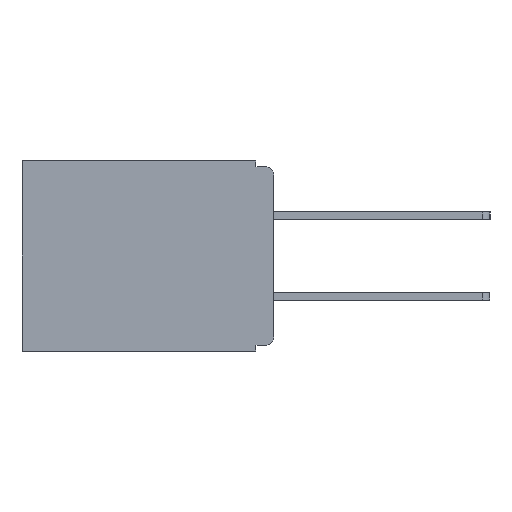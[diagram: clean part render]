
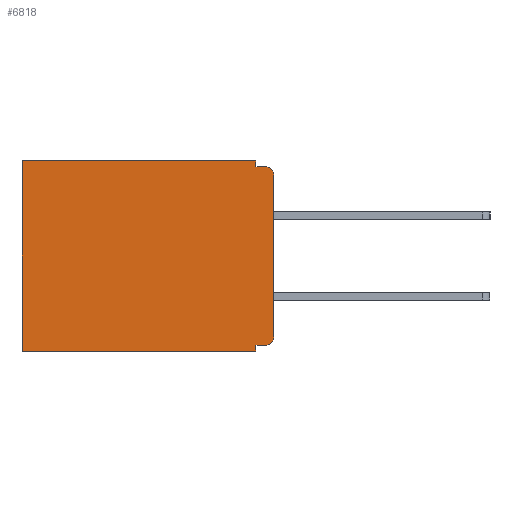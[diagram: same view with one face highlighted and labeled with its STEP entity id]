
A CAD part, left-side view. The second image highlights one B-rep face of the part: STEP entity #6818.
In plain terms, the highlighted planar face has unit normal (-1, 0, 0).
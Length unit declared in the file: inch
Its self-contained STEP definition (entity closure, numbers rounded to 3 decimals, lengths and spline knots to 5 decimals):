
#93 = DIRECTION ( 'NONE',  ( 1., 0., 0. ) ) ;
#342 = VECTOR ( 'NONE', #3753, 39.37008 ) ;
#639 = ORIENTED_EDGE ( 'NONE', *, *, #15581, .T. ) ;
#849 = VECTOR ( 'NONE', #10346, 39.37008 ) ;
#1255 = EDGE_CURVE ( 'NONE', #26265, #23395, #8771, .T. ) ;
#1268 = EDGE_CURVE ( 'NONE', #26265, #24596, #8109, .T. ) ;
#1290 = CARTESIAN_POINT ( 'NONE',  ( 0.3, 0.437, -0.33 ) ) ;
#1765 = VERTEX_POINT ( 'NONE', #7767 ) ;
#1781 = CARTESIAN_POINT ( 'NONE',  ( 0.3, 0.015, -0.305 ) ) ;
#1952 = VERTEX_POINT ( 'NONE', #24529 ) ;
#1975 = ORIENTED_EDGE ( 'NONE', *, *, #1268, .F. ) ;
#1980 = EDGE_CURVE ( 'NONE', #24596, #8565, #9445, .T. ) ;
#2009 = ORIENTED_EDGE ( 'NONE', *, *, #17366, .T. ) ;
#3186 = PLANE ( 'NONE',  #14296 ) ;
#3435 = VERTEX_POINT ( 'NONE', #1290 ) ;
#3664 = VECTOR ( 'NONE', #17647, 39.37008 ) ;
#3705 = DIRECTION ( 'NONE',  ( -1., 0., 0. ) ) ;
#3753 = DIRECTION ( 'NONE',  ( 0., 0., -1. ) ) ;
#4044 = DIRECTION ( 'NONE',  ( 0., 0., -1. ) ) ;
#4134 = VERTEX_POINT ( 'NONE', #11212 ) ;
#4178 = AXIS2_PLACEMENT_3D ( 'NONE', #1781, #16551, #4044 ) ;
#4761 = CARTESIAN_POINT ( 'NONE',  ( 0.3, 0., -0.01 ) ) ;
#4827 = CARTESIAN_POINT ( 'NONE',  ( 0.3, 0.015, -0.32 ) ) ;
#5767 = DIRECTION ( 'NONE',  ( 0., 0., -1. ) ) ;
#6818 = ADVANCED_FACE ( 'NONE', ( #14408 ), #3186, .F. ) ;
#7631 = DIRECTION ( 'NONE',  ( 0., 0., -1. ) ) ;
#7641 = ORIENTED_EDGE ( 'NONE', *, *, #15970, .F. ) ;
#7767 = CARTESIAN_POINT ( 'NONE',  ( 0.3, 0., -0.305 ) ) ;
#8109 = LINE ( 'NONE', #25941, #14249 ) ;
#8565 = VERTEX_POINT ( 'NONE', #25086 ) ;
#8660 = ORIENTED_EDGE ( 'NONE', *, *, #1980, .F. ) ;
#8670 = LINE ( 'NONE', #21833, #18209 ) ;
#8771 = LINE ( 'NONE', #24153, #13592 ) ;
#9291 = LINE ( 'NONE', #22622, #20660 ) ;
#9384 = ORIENTED_EDGE ( 'NONE', *, *, #19107, .F. ) ;
#9434 = ORIENTED_EDGE ( 'NONE', *, *, #25076, .F. ) ;
#9445 = LINE ( 'NONE', #4761, #3664 ) ;
#10346 = DIRECTION ( 'NONE',  ( 0., 1., 0. ) ) ;
#11212 = CARTESIAN_POINT ( 'NONE',  ( 0.3, 0., -0.025 ) ) ;
#11640 = LINE ( 'NONE', #22080, #26401 ) ;
#12965 = ORIENTED_EDGE ( 'NONE', *, *, #14863, .T. ) ;
#13592 = VECTOR ( 'NONE', #25249, 39.37008 ) ;
#14249 = VECTOR ( 'NONE', #25065, 39.37008 ) ;
#14296 = AXIS2_PLACEMENT_3D ( 'NONE', #24427, #93, #7631 ) ;
#14314 = EDGE_CURVE ( 'NONE', #1952, #3435, #17671, .T. ) ;
#14408 = FACE_OUTER_BOUND ( 'NONE', #26288, .T. ) ;
#14529 = CIRCLE ( 'NONE', #15588, 0.015 ) ;
#14863 = EDGE_CURVE ( 'NONE', #4134, #8565, #14529, .T. ) ;
#15581 = EDGE_CURVE ( 'NONE', #17558, #1765, #18234, .T. ) ;
#15588 = AXIS2_PLACEMENT_3D ( 'NONE', #16240, #3705, #18256 ) ;
#15970 = EDGE_CURVE ( 'NONE', #17558, #24839, #8670, .T. ) ;
#16240 = CARTESIAN_POINT ( 'NONE',  ( 0.3, 0.015, -0.025 ) ) ;
#16551 = DIRECTION ( 'NONE',  ( -1., 0., 0. ) ) ;
#17366 = EDGE_CURVE ( 'NONE', #23395, #3435, #9291, .T. ) ;
#17558 = VERTEX_POINT ( 'NONE', #4827 ) ;
#17647 = DIRECTION ( 'NONE',  ( 0., -1., 0. ) ) ;
#17671 = LINE ( 'NONE', #18374, #849 ) ;
#17851 = LINE ( 'NONE', #20300, #342 ) ;
#18209 = VECTOR ( 'NONE', #23870, 39.37008 ) ;
#18234 = CIRCLE ( 'NONE', #4178, 0.015 ) ;
#18256 = DIRECTION ( 'NONE',  ( 0., 0., -1. ) ) ;
#18374 = CARTESIAN_POINT ( 'NONE',  ( 0.3, 0., -0.33 ) ) ;
#18924 = CARTESIAN_POINT ( 'NONE',  ( 0.3, 0.437, 0. ) ) ;
#18957 = CARTESIAN_POINT ( 'NONE',  ( 0.3, 0.031, -0.01 ) ) ;
#19107 = EDGE_CURVE ( 'NONE', #4134, #1765, #17851, .T. ) ;
#20300 = CARTESIAN_POINT ( 'NONE',  ( 0.3, 0., -0.33 ) ) ;
#20660 = VECTOR ( 'NONE', #24697, 39.37008 ) ;
#21293 = ORIENTED_EDGE ( 'NONE', *, *, #1255, .T. ) ;
#21833 = CARTESIAN_POINT ( 'NONE',  ( 0.3, 0., -0.32 ) ) ;
#22080 = CARTESIAN_POINT ( 'NONE',  ( 0.3, 0.031, -0.33 ) ) ;
#22622 = CARTESIAN_POINT ( 'NONE',  ( 0.3, 0.437, -0.33 ) ) ;
#23275 = ORIENTED_EDGE ( 'NONE', *, *, #14314, .F. ) ;
#23395 = VERTEX_POINT ( 'NONE', #18924 ) ;
#23870 = DIRECTION ( 'NONE',  ( 0., 1., 0. ) ) ;
#23972 = CARTESIAN_POINT ( 'NONE',  ( 0.3, 0.031, 0. ) ) ;
#24153 = CARTESIAN_POINT ( 'NONE',  ( 0.3, 0., 0. ) ) ;
#24427 = CARTESIAN_POINT ( 'NONE',  ( 0.3, 0., -0.33 ) ) ;
#24529 = CARTESIAN_POINT ( 'NONE',  ( 0.3, 0.031, -0.33 ) ) ;
#24596 = VERTEX_POINT ( 'NONE', #18957 ) ;
#24697 = DIRECTION ( 'NONE',  ( 0., 0., -1. ) ) ;
#24839 = VERTEX_POINT ( 'NONE', #25697 ) ;
#25065 = DIRECTION ( 'NONE',  ( 0., 0., -1. ) ) ;
#25076 = EDGE_CURVE ( 'NONE', #24839, #1952, #11640, .T. ) ;
#25086 = CARTESIAN_POINT ( 'NONE',  ( 0.3, 0.015, -0.01 ) ) ;
#25249 = DIRECTION ( 'NONE',  ( 0., 1., 0. ) ) ;
#25697 = CARTESIAN_POINT ( 'NONE',  ( 0.3, 0.031, -0.32 ) ) ;
#25941 = CARTESIAN_POINT ( 'NONE',  ( 0.3, 0.031, 0. ) ) ;
#26265 = VERTEX_POINT ( 'NONE', #23972 ) ;
#26288 = EDGE_LOOP ( 'NONE', ( #9384, #12965, #8660, #1975, #21293, #2009, #23275, #9434, #7641, #639 ) ) ;
#26401 = VECTOR ( 'NONE', #5767, 39.37008 ) ;
